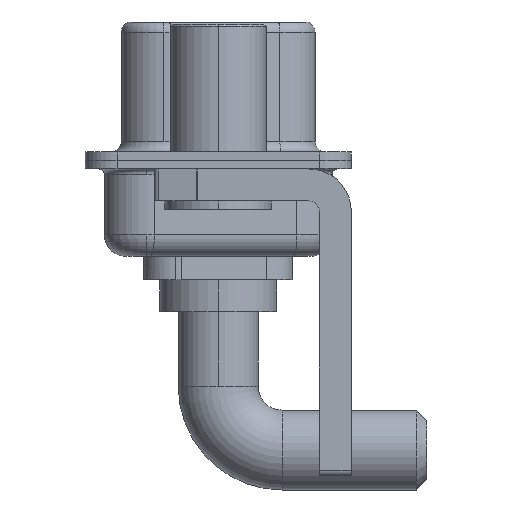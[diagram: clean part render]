
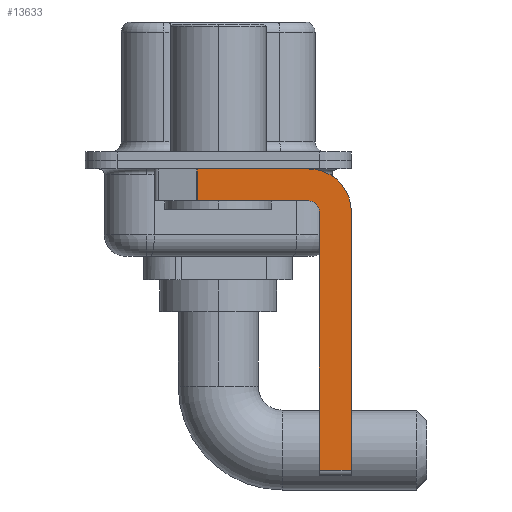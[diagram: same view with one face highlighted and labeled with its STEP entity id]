
A CAD part, left-side view. The second image highlights one B-rep face of the part: STEP entity #13633.
In plain terms, the highlighted planar face has unit normal (-1, 0, 0).
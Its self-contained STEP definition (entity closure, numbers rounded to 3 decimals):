
#19 = DIRECTION ( 'NONE',  ( 0., 0., -1. ) ) ;
#189 = LINE ( 'NONE', #5227, #13381 ) ;
#198 = VERTEX_POINT ( 'NONE', #14955 ) ;
#387 = AXIS2_PLACEMENT_3D ( 'NONE', #11172, #8174, #5607 ) ;
#598 = VERTEX_POINT ( 'NONE', #7921 ) ;
#599 = ORIENTED_EDGE ( 'NONE', *, *, #8009, .F. ) ;
#636 = PLANE ( 'NONE',  #12385 ) ;
#1721 = VECTOR ( 'NONE', #12602, 1000. ) ;
#1724 = ORIENTED_EDGE ( 'NONE', *, *, #2745, .F. ) ;
#1853 = VERTEX_POINT ( 'NONE', #4659 ) ;
#1891 = EDGE_CURVE ( 'NONE', #1853, #11012, #4407, .T. ) ;
#2493 = EDGE_CURVE ( 'NONE', #12548, #4747, #189, .T. ) ;
#2537 = ORIENTED_EDGE ( 'NONE', *, *, #9783, .F. ) ;
#2745 = EDGE_CURVE ( 'NONE', #198, #598, #5181, .T. ) ;
#3086 = CARTESIAN_POINT ( 'NONE',  ( -2.9, -4.25, -2.4 ) ) ;
#3526 = LINE ( 'NONE', #15171, #1721 ) ;
#3563 = EDGE_CURVE ( 'NONE', #12548, #198, #9866, .T. ) ;
#3582 = EDGE_CURVE ( 'NONE', #15261, #4747, #3526, .T. ) ;
#3632 = VECTOR ( 'NONE', #4635, 1000. ) ;
#4407 = LINE ( 'NONE', #13262, #11968 ) ;
#4573 = DIRECTION ( 'NONE',  ( 0., -1., 0. ) ) ;
#4635 = DIRECTION ( 'NONE',  ( 0., -1., 0. ) ) ;
#4659 = CARTESIAN_POINT ( 'NONE',  ( -2.9, -4.75, -14.55 ) ) ;
#4747 = VERTEX_POINT ( 'NONE', #10327 ) ;
#4952 = EDGE_CURVE ( 'NONE', #6916, #15261, #15147, .T. ) ;
#5181 = CIRCLE ( 'NONE', #14206, 2. ) ;
#5227 = CARTESIAN_POINT ( 'NONE',  ( -2.9, 0.978, -1.9 ) ) ;
#5607 = DIRECTION ( 'NONE',  ( 0., 0., 1. ) ) ;
#6488 = CARTESIAN_POINT ( 'NONE',  ( -2.9, -4.75, -2.4 ) ) ;
#6496 = LINE ( 'NONE', #14380, #15887 ) ;
#6549 = VECTOR ( 'NONE', #7003, 1000. ) ;
#6613 = ORIENTED_EDGE ( 'NONE', *, *, #2493, .T. ) ;
#6916 = VERTEX_POINT ( 'NONE', #6488 ) ;
#7003 = DIRECTION ( 'NONE',  ( 0., 0., -1. ) ) ;
#7205 = DIRECTION ( 'NONE',  ( 1., 0., 0. ) ) ;
#7458 = CARTESIAN_POINT ( 'NONE',  ( -2.9, 3., -0.4 ) ) ;
#7921 = CARTESIAN_POINT ( 'NONE',  ( -2.9, -6.25, -2.4 ) ) ;
#8009 = EDGE_CURVE ( 'NONE', #598, #11012, #8375, .T. ) ;
#8174 = DIRECTION ( 'NONE',  ( -1., 0., 0. ) ) ;
#8220 = ORIENTED_EDGE ( 'NONE', *, *, #3582, .F. ) ;
#8375 = LINE ( 'NONE', #11979, #6549 ) ;
#9704 = ORIENTED_EDGE ( 'NONE', *, *, #4952, .F. ) ;
#9783 = EDGE_CURVE ( 'NONE', #1853, #6916, #6496, .T. ) ;
#9866 = LINE ( 'NONE', #7458, #3632 ) ;
#10327 = CARTESIAN_POINT ( 'NONE',  ( -2.9, 0.978, -1.9 ) ) ;
#10903 = EDGE_LOOP ( 'NONE', ( #13167, #6613, #8220, #9704, #2537, #16828, #599, #1724 ) ) ;
#11012 = VERTEX_POINT ( 'NONE', #16545 ) ;
#11172 = CARTESIAN_POINT ( 'NONE',  ( -2.9, -4.25, -2.4 ) ) ;
#11968 = VECTOR ( 'NONE', #4573, 1000. ) ;
#11979 = CARTESIAN_POINT ( 'NONE',  ( -2.9, -6.25, -2.4 ) ) ;
#12154 = DIRECTION ( 'NONE',  ( 1., 0., 0. ) ) ;
#12326 = DIRECTION ( 'NONE',  ( 0., 0., -1. ) ) ;
#12351 = FACE_OUTER_BOUND ( 'NONE', #10903, .T. ) ;
#12385 = AXIS2_PLACEMENT_3D ( 'NONE', #13466, #7205, #14746 ) ;
#12548 = VERTEX_POINT ( 'NONE', #15601 ) ;
#12602 = DIRECTION ( 'NONE',  ( 0., 1., 0. ) ) ;
#13087 = DIRECTION ( 'NONE',  ( 0., 0., 1. ) ) ;
#13167 = ORIENTED_EDGE ( 'NONE', *, *, #3563, .F. ) ;
#13262 = CARTESIAN_POINT ( 'NONE',  ( -2.9, -4.25, -14.55 ) ) ;
#13381 = VECTOR ( 'NONE', #19, 1000. ) ;
#13466 = CARTESIAN_POINT ( 'NONE',  ( -2.9, -4.25, -2.4 ) ) ;
#13633 = ADVANCED_FACE ( 'NONE', ( #12351 ), #636, .F. ) ;
#14206 = AXIS2_PLACEMENT_3D ( 'NONE', #3086, #12154, #12326 ) ;
#14380 = CARTESIAN_POINT ( 'NONE',  ( -2.9, -4.75, -14.8 ) ) ;
#14746 = DIRECTION ( 'NONE',  ( 0., 0., -1. ) ) ;
#14955 = CARTESIAN_POINT ( 'NONE',  ( -2.9, -4.25, -0.4 ) ) ;
#15147 = CIRCLE ( 'NONE', #387, 0.5 ) ;
#15171 = CARTESIAN_POINT ( 'NONE',  ( -2.9, -4.25, -1.9 ) ) ;
#15261 = VERTEX_POINT ( 'NONE', #15960 ) ;
#15601 = CARTESIAN_POINT ( 'NONE',  ( -2.9, 0.978, -0.4 ) ) ;
#15887 = VECTOR ( 'NONE', #13087, 1000. ) ;
#15960 = CARTESIAN_POINT ( 'NONE',  ( -2.9, -4.25, -1.9 ) ) ;
#16545 = CARTESIAN_POINT ( 'NONE',  ( -2.9, -6.25, -14.55 ) ) ;
#16828 = ORIENTED_EDGE ( 'NONE', *, *, #1891, .T. ) ;
